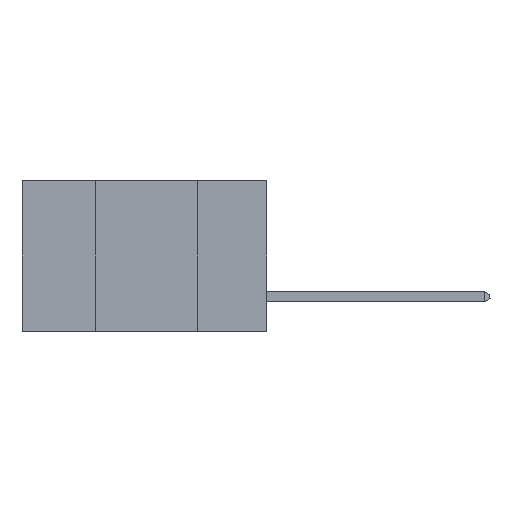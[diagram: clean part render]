
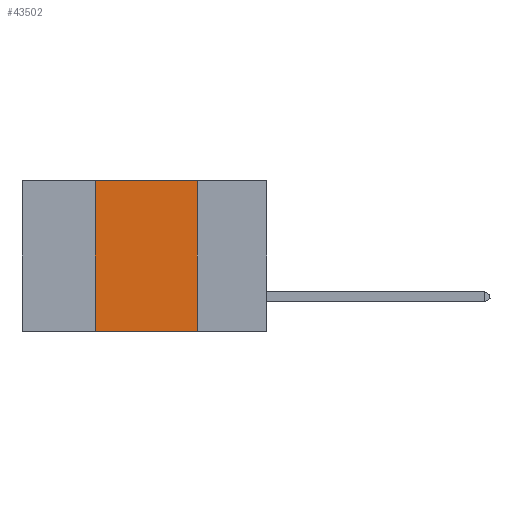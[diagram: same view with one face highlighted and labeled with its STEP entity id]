
A CAD part, left-side view. The second image highlights one B-rep face of the part: STEP entity #43502.
In plain terms, the highlighted planar face has unit normal (-1, 0, 0).
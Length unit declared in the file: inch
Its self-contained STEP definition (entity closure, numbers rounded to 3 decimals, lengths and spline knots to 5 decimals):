
#211 = FACE_OUTER_BOUND ( 'NONE', #29767, .T. ) ;
#2474 = CARTESIAN_POINT ( 'NONE',  ( 0., 0.17, -0.37 ) ) ;
#4235 = LINE ( 'NONE', #24352, #35210 ) ;
#4479 = DIRECTION ( 'NONE',  ( 0., -1., 0. ) ) ;
#4968 = CARTESIAN_POINT ( 'NONE',  ( 0., 0.17, 0. ) ) ;
#7406 = DIRECTION ( 'NONE',  ( 0., 0., -1. ) ) ;
#8262 = LINE ( 'NONE', #4968, #39813 ) ;
#8399 = CARTESIAN_POINT ( 'NONE',  ( 0., 0.6, -0.37 ) ) ;
#8534 = VECTOR ( 'NONE', #4479, 39.37008 ) ;
#8798 = CARTESIAN_POINT ( 'NONE',  ( 0., 0.17, 0. ) ) ;
#9772 = CARTESIAN_POINT ( 'NONE',  ( 0., 0.42, -0.37 ) ) ;
#12281 = DIRECTION ( 'NONE',  ( 0., -1., 0. ) ) ;
#14734 = VERTEX_POINT ( 'NONE', #8798 ) ;
#15454 = LINE ( 'NONE', #40839, #22715 ) ;
#17600 = EDGE_CURVE ( 'NONE', #39665, #19416, #15454, .T. ) ;
#18951 = PLANE ( 'NONE',  #49776 ) ;
#19416 = VERTEX_POINT ( 'NONE', #30076 ) ;
#21138 = VERTEX_POINT ( 'NONE', #2474 ) ;
#22715 = VECTOR ( 'NONE', #48486, 39.37008 ) ;
#22771 = EDGE_CURVE ( 'NONE', #39665, #21138, #26108, .T. ) ;
#22840 = EDGE_CURVE ( 'NONE', #19416, #14734, #4235, .T. ) ;
#24352 = CARTESIAN_POINT ( 'NONE',  ( 0., 0.6, 0. ) ) ;
#26108 = LINE ( 'NONE', #8399, #8534 ) ;
#26509 = ORIENTED_EDGE ( 'NONE', *, *, #22840, .F. ) ;
#27242 = ORIENTED_EDGE ( 'NONE', *, *, #17600, .F. ) ;
#29767 = EDGE_LOOP ( 'NONE', ( #32104, #26509, #27242, #37329 ) ) ;
#30076 = CARTESIAN_POINT ( 'NONE',  ( 0., 0.42, 0. ) ) ;
#32104 = ORIENTED_EDGE ( 'NONE', *, *, #42520, .F. ) ;
#34233 = CARTESIAN_POINT ( 'NONE',  ( 0., 0.6, 0. ) ) ;
#35210 = VECTOR ( 'NONE', #12281, 39.37008 ) ;
#36980 = DIRECTION ( 'NONE',  ( 0., 0., -1. ) ) ;
#37329 = ORIENTED_EDGE ( 'NONE', *, *, #22771, .T. ) ;
#39665 = VERTEX_POINT ( 'NONE', #9772 ) ;
#39813 = VECTOR ( 'NONE', #36980, 39.37008 ) ;
#40839 = CARTESIAN_POINT ( 'NONE',  ( 0., 0.42, 0. ) ) ;
#42520 = EDGE_CURVE ( 'NONE', #14734, #21138, #8262, .T. ) ;
#43502 = ADVANCED_FACE ( 'NONE', ( #211 ), #18951, .F. ) ;
#46258 = DIRECTION ( 'NONE',  ( 1., 0., 0. ) ) ;
#48486 = DIRECTION ( 'NONE',  ( 0., 0., 1. ) ) ;
#49776 = AXIS2_PLACEMENT_3D ( 'NONE', #34233, #46258, #7406 ) ;
